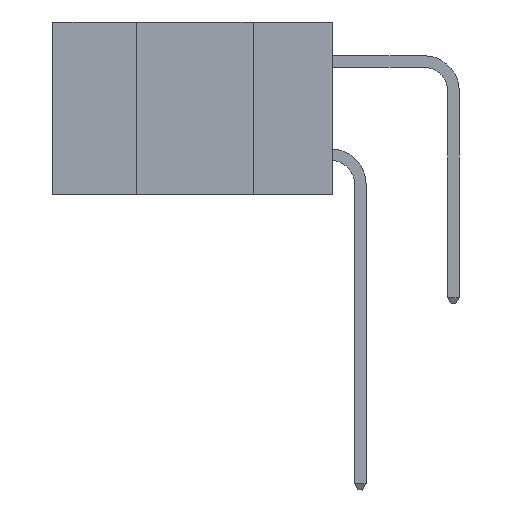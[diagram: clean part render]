
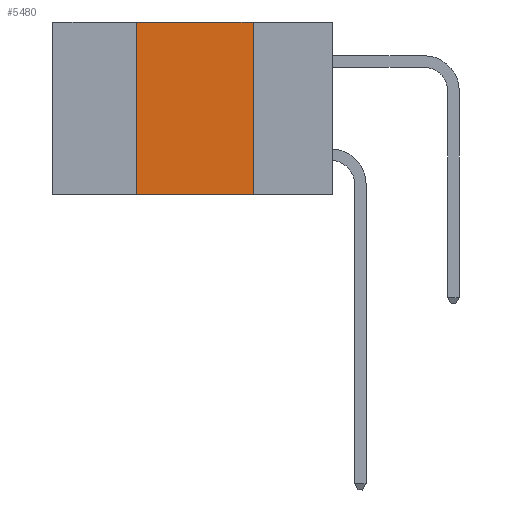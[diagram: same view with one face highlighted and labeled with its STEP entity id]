
A CAD part, left-side view. The second image highlights one B-rep face of the part: STEP entity #5480.
In plain terms, the highlighted planar face has unit normal (-1, 0, 0).
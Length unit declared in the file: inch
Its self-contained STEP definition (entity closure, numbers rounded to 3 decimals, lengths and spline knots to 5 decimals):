
#551 = ORIENTED_EDGE ( 'NONE', *, *, #4621, .F. ) ;
#1970 = CARTESIAN_POINT ( 'NONE',  ( 0., 0.6, 0. ) ) ;
#2813 = ORIENTED_EDGE ( 'NONE', *, *, #13575, .T. ) ;
#2821 = VERTEX_POINT ( 'NONE', #3946 ) ;
#3277 = LINE ( 'NONE', #12097, #10512 ) ;
#3781 = DIRECTION ( 'NONE',  ( 0., 0., -1. ) ) ;
#3813 = DIRECTION ( 'NONE',  ( 0., -1., 0. ) ) ;
#3912 = DIRECTION ( 'NONE',  ( 1., 0., 0. ) ) ;
#3946 = CARTESIAN_POINT ( 'NONE',  ( 0., 0.17, 0. ) ) ;
#3978 = PLANE ( 'NONE',  #18229 ) ;
#4159 = CARTESIAN_POINT ( 'NONE',  ( 0., 0.6, 0. ) ) ;
#4621 = EDGE_CURVE ( 'NONE', #7775, #15988, #3277, .T. ) ;
#5480 = ADVANCED_FACE ( 'NONE', ( #7075 ), #3978, .F. ) ;
#5667 = ORIENTED_EDGE ( 'NONE', *, *, #10414, .F. ) ;
#7036 = CARTESIAN_POINT ( 'NONE',  ( 0., 0.42, 0. ) ) ;
#7075 = FACE_OUTER_BOUND ( 'NONE', #7704, .T. ) ;
#7704 = EDGE_LOOP ( 'NONE', ( #5667, #8196, #551, #2813 ) ) ;
#7775 = VERTEX_POINT ( 'NONE', #12326 ) ;
#8196 = ORIENTED_EDGE ( 'NONE', *, *, #14021, .F. ) ;
#9564 = CARTESIAN_POINT ( 'NONE',  ( 0., 0.6, -0.37 ) ) ;
#10343 = VERTEX_POINT ( 'NONE', #14011 ) ;
#10414 = EDGE_CURVE ( 'NONE', #2821, #10343, #11662, .T. ) ;
#10512 = VECTOR ( 'NONE', #11524, 39.37008 ) ;
#10891 = LINE ( 'NONE', #1970, #14966 ) ;
#10905 = VECTOR ( 'NONE', #3813, 39.37008 ) ;
#11524 = DIRECTION ( 'NONE',  ( 0., 0., 1. ) ) ;
#11662 = LINE ( 'NONE', #16833, #14855 ) ;
#12023 = DIRECTION ( 'NONE',  ( 0., -1., 0. ) ) ;
#12097 = CARTESIAN_POINT ( 'NONE',  ( 0., 0.42, 0. ) ) ;
#12326 = CARTESIAN_POINT ( 'NONE',  ( 0., 0.42, -0.37 ) ) ;
#13575 = EDGE_CURVE ( 'NONE', #7775, #10343, #14979, .T. ) ;
#14011 = CARTESIAN_POINT ( 'NONE',  ( 0., 0.17, -0.37 ) ) ;
#14021 = EDGE_CURVE ( 'NONE', #15988, #2821, #10891, .T. ) ;
#14855 = VECTOR ( 'NONE', #18180, 39.37008 ) ;
#14966 = VECTOR ( 'NONE', #12023, 39.37008 ) ;
#14979 = LINE ( 'NONE', #9564, #10905 ) ;
#15988 = VERTEX_POINT ( 'NONE', #7036 ) ;
#16833 = CARTESIAN_POINT ( 'NONE',  ( 0., 0.17, 0. ) ) ;
#18180 = DIRECTION ( 'NONE',  ( 0., 0., -1. ) ) ;
#18229 = AXIS2_PLACEMENT_3D ( 'NONE', #4159, #3912, #3781 ) ;
